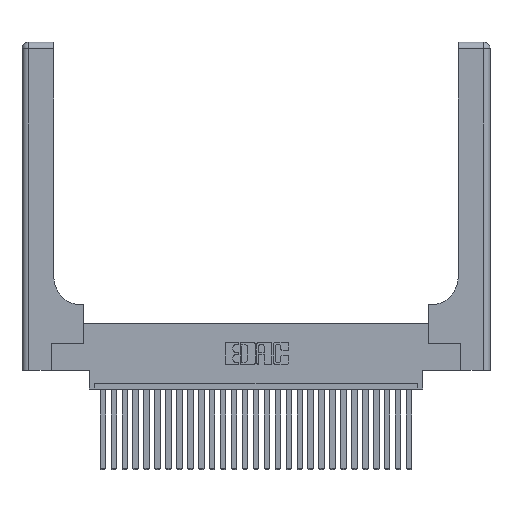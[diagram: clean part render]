
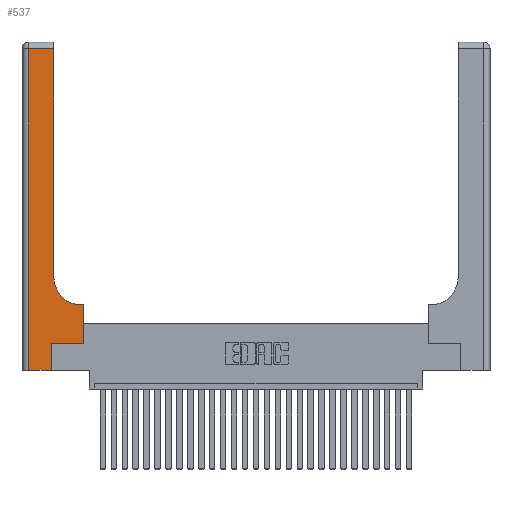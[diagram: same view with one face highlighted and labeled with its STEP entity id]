
A CAD part, top view. The second image highlights one B-rep face of the part: STEP entity #537.
In plain terms, the highlighted planar face has unit normal (0, 0, 1).
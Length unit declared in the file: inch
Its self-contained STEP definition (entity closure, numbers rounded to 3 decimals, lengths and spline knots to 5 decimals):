
#195 = VECTOR ( 'NONE', #15959, 39.37008 ) ;
#537 = ADVANCED_FACE ( 'NONE', ( #8470 ), #26308, .F. ) ;
#773 = ORIENTED_EDGE ( 'NONE', *, *, #10005, .T. ) ;
#994 = DIRECTION ( 'NONE',  ( -1., 0., 0. ) ) ;
#1088 = VECTOR ( 'NONE', #6601, 39.37008 ) ;
#1473 = LINE ( 'NONE', #15106, #24389 ) ;
#2112 = CARTESIAN_POINT ( 'NONE',  ( 0.269, 0.25, 0.37 ) ) ;
#2240 = VERTEX_POINT ( 'NONE', #18194 ) ;
#2333 = EDGE_CURVE ( 'NONE', #15033, #26611, #4517, .T. ) ;
#2648 = ORIENTED_EDGE ( 'NONE', *, *, #27199, .T. ) ;
#3155 = ORIENTED_EDGE ( 'NONE', *, *, #19748, .T. ) ;
#3301 = CARTESIAN_POINT ( 'NONE',  ( 0.5415, 0.6, 0.37 ) ) ;
#3887 = VERTEX_POINT ( 'NONE', #2112 ) ;
#3967 = DIRECTION ( 'NONE',  ( 1., 0., 0. ) ) ;
#4249 = CARTESIAN_POINT ( 'NONE',  ( 0.269, 0., 0.37 ) ) ;
#4267 = DIRECTION ( 'NONE',  ( 0., 0., -1. ) ) ;
#4278 = LINE ( 'NONE', #19664, #17430 ) ;
#4517 = LINE ( 'NONE', #22543, #1088 ) ;
#4588 = VERTEX_POINT ( 'NONE', #14268 ) ;
#4838 = CIRCLE ( 'NONE', #20429, 0.25 ) ;
#5116 = VERTEX_POINT ( 'NONE', #3301 ) ;
#5352 = CARTESIAN_POINT ( 'NONE',  ( 0.2915, 2.94, 0.37 ) ) ;
#6086 = DIRECTION ( 'NONE',  ( 0., 1., 0. ) ) ;
#6376 = DIRECTION ( 'NONE',  ( -1., 0., 0. ) ) ;
#6601 = DIRECTION ( 'NONE',  ( 0., -1., 0. ) ) ;
#6842 = CARTESIAN_POINT ( 'NONE',  ( 0.269, 0., 0.37 ) ) ;
#7890 = ORIENTED_EDGE ( 'NONE', *, *, #15760, .T. ) ;
#8470 = FACE_OUTER_BOUND ( 'NONE', #19919, .T. ) ;
#8623 = EDGE_CURVE ( 'NONE', #5116, #4588, #4838, .T. ) ;
#9614 = CARTESIAN_POINT ( 'NONE',  ( 0.5415, 0.85, 0.37 ) ) ;
#9794 = CARTESIAN_POINT ( 'NONE',  ( 0., 2.94, 0.37 ) ) ;
#9919 = DIRECTION ( 'NONE',  ( 0., 0., -1. ) ) ;
#10005 = EDGE_CURVE ( 'NONE', #16315, #3887, #20678, .T. ) ;
#10048 = LINE ( 'NONE', #24690, #27651 ) ;
#11202 = ORIENTED_EDGE ( 'NONE', *, *, #24458, .T. ) ;
#11621 = CARTESIAN_POINT ( 'NONE',  ( 0.06, 0., 0.37 ) ) ;
#11730 = DIRECTION ( 'NONE',  ( -1., 0., 0. ) ) ;
#11771 = CARTESIAN_POINT ( 'NONE',  ( 0.2915, 3., 0.37 ) ) ;
#12319 = EDGE_CURVE ( 'NONE', #2240, #24488, #1473, .T. ) ;
#13207 = ORIENTED_EDGE ( 'NONE', *, *, #2333, .T. ) ;
#13494 = DIRECTION ( 'NONE',  ( 0., 1., 0. ) ) ;
#13612 = CARTESIAN_POINT ( 'NONE',  ( 0.5585, 0.6, 0.37 ) ) ;
#13786 = ORIENTED_EDGE ( 'NONE', *, *, #27887, .T. ) ;
#14268 = CARTESIAN_POINT ( 'NONE',  ( 0.2915, 0.85, 0.37 ) ) ;
#14502 = AXIS2_PLACEMENT_3D ( 'NONE', #15028, #4267, #6376 ) ;
#14562 = DIRECTION ( 'NONE',  ( 1., 0., 0. ) ) ;
#15028 = CARTESIAN_POINT ( 'NONE',  ( 0., 3., 0.37 ) ) ;
#15033 = VERTEX_POINT ( 'NONE', #21021 ) ;
#15106 = CARTESIAN_POINT ( 'NONE',  ( 0.5585, 0.25, 0.37 ) ) ;
#15760 = EDGE_CURVE ( 'NONE', #26611, #16315, #10048, .T. ) ;
#15959 = DIRECTION ( 'NONE',  ( 0., 1., 0. ) ) ;
#16315 = VERTEX_POINT ( 'NONE', #4249 ) ;
#17430 = VECTOR ( 'NONE', #3967, 39.37008 ) ;
#17587 = VECTOR ( 'NONE', #13494, 39.37008 ) ;
#18194 = CARTESIAN_POINT ( 'NONE',  ( 0.5585, 0.25, 0.37 ) ) ;
#18451 = VECTOR ( 'NONE', #11730, 39.37008 ) ;
#19664 = CARTESIAN_POINT ( 'NONE',  ( 0.269, 0.25, 0.37 ) ) ;
#19748 = EDGE_CURVE ( 'NONE', #24488, #5116, #24392, .T. ) ;
#19919 = EDGE_LOOP ( 'NONE', ( #2648, #13786, #13207, #7890, #773, #11202, #25835, #3155, #20952 ) ) ;
#20429 = AXIS2_PLACEMENT_3D ( 'NONE', #9614, #9919, #14562 ) ;
#20477 = CARTESIAN_POINT ( 'NONE',  ( 0.2915, 0.6, 0.37 ) ) ;
#20678 = LINE ( 'NONE', #6842, #195 ) ;
#20952 = ORIENTED_EDGE ( 'NONE', *, *, #8623, .T. ) ;
#21021 = CARTESIAN_POINT ( 'NONE',  ( 0.06, 2.94, 0.37 ) ) ;
#21122 = LINE ( 'NONE', #11771, #17587 ) ;
#22543 = CARTESIAN_POINT ( 'NONE',  ( 0.06, 3., 0.37 ) ) ;
#23168 = LINE ( 'NONE', #9794, #25234 ) ;
#24389 = VECTOR ( 'NONE', #6086, 39.37008 ) ;
#24392 = LINE ( 'NONE', #20477, #18451 ) ;
#24458 = EDGE_CURVE ( 'NONE', #3887, #2240, #4278, .T. ) ;
#24488 = VERTEX_POINT ( 'NONE', #13612 ) ;
#24690 = CARTESIAN_POINT ( 'NONE',  ( 0., 0., 0.37 ) ) ;
#25234 = VECTOR ( 'NONE', #994, 39.37008 ) ;
#25403 = VERTEX_POINT ( 'NONE', #5352 ) ;
#25835 = ORIENTED_EDGE ( 'NONE', *, *, #12319, .T. ) ;
#26308 = PLANE ( 'NONE',  #14502 ) ;
#26611 = VERTEX_POINT ( 'NONE', #11621 ) ;
#26997 = DIRECTION ( 'NONE',  ( 1., 0., 0. ) ) ;
#27199 = EDGE_CURVE ( 'NONE', #4588, #25403, #21122, .T. ) ;
#27651 = VECTOR ( 'NONE', #26997, 39.37008 ) ;
#27887 = EDGE_CURVE ( 'NONE', #25403, #15033, #23168, .T. ) ;
